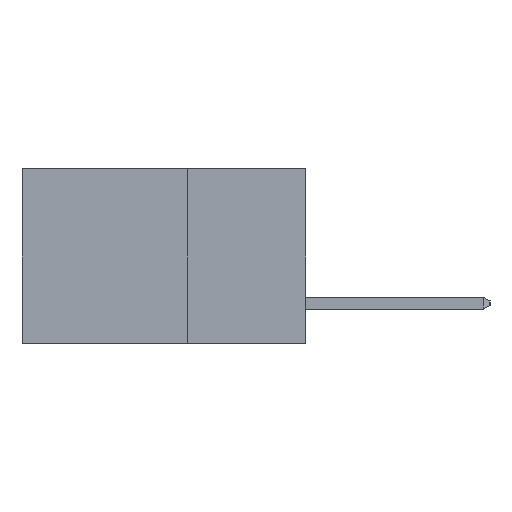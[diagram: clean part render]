
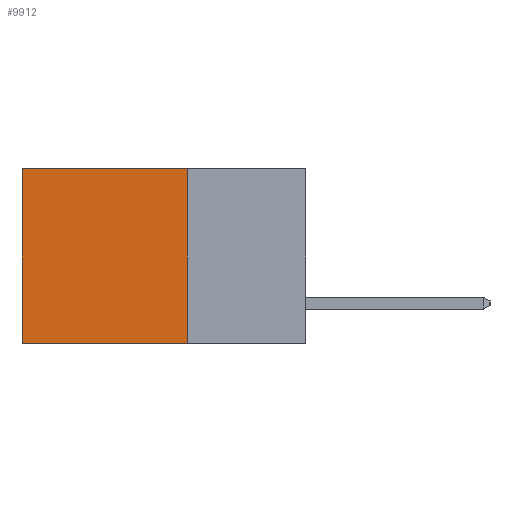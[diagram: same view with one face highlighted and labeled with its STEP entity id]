
A CAD part, left-side view. The second image highlights one B-rep face of the part: STEP entity #9912.
In plain terms, the highlighted planar face has unit normal (-1, 0, 0).
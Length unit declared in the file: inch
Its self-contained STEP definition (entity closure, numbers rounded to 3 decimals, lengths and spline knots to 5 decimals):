
#620 = LINE ( 'NONE', #13677, #1157 ) ;
#1157 = VECTOR ( 'NONE', #13656, 39.37008 ) ;
#1294 = LINE ( 'NONE', #17770, #9365 ) ;
#1515 = DIRECTION ( 'NONE',  ( 0., 1., 0. ) ) ;
#1971 = CARTESIAN_POINT ( 'NONE',  ( 0.2615, 0.6, 0. ) ) ;
#2128 = CARTESIAN_POINT ( 'NONE',  ( 0.2615, 0.25, -0.37 ) ) ;
#2547 = VERTEX_POINT ( 'NONE', #5227 ) ;
#4228 = ORIENTED_EDGE ( 'NONE', *, *, #6359, .F. ) ;
#5227 = CARTESIAN_POINT ( 'NONE',  ( 0.2615, 0.6, -0.37 ) ) ;
#5996 = VECTOR ( 'NONE', #1515, 39.37008 ) ;
#6359 = EDGE_CURVE ( 'NONE', #9627, #2547, #15925, .T. ) ;
#6627 = VERTEX_POINT ( 'NONE', #16315 ) ;
#9365 = VECTOR ( 'NONE', #17701, 39.37008 ) ;
#9627 = VERTEX_POINT ( 'NONE', #17971 ) ;
#9912 = ADVANCED_FACE ( 'NONE', ( #15839 ), #18465, .F. ) ;
#10408 = EDGE_CURVE ( 'NONE', #6627, #9627, #15329, .T. ) ;
#11313 = EDGE_CURVE ( 'NONE', #6627, #17064, #1294, .T. ) ;
#11904 = ORIENTED_EDGE ( 'NONE', *, *, #11313, .T. ) ;
#12364 = AXIS2_PLACEMENT_3D ( 'NONE', #18436, #18370, #18341 ) ;
#12371 = ORIENTED_EDGE ( 'NONE', *, *, #14330, .T. ) ;
#13656 = DIRECTION ( 'NONE',  ( 0., 0., -1. ) ) ;
#13677 = CARTESIAN_POINT ( 'NONE',  ( 0.2615, 0.6, -0.37 ) ) ;
#14330 = EDGE_CURVE ( 'NONE', #17064, #2547, #620, .T. ) ;
#14795 = EDGE_LOOP ( 'NONE', ( #12371, #4228, #17617, #11904 ) ) ;
#15329 = LINE ( 'NONE', #20101, #18571 ) ;
#15839 = FACE_OUTER_BOUND ( 'NONE', #14795, .T. ) ;
#15925 = LINE ( 'NONE', #2128, #5996 ) ;
#16315 = CARTESIAN_POINT ( 'NONE',  ( 0.2615, 0.25, 0. ) ) ;
#17064 = VERTEX_POINT ( 'NONE', #1971 ) ;
#17617 = ORIENTED_EDGE ( 'NONE', *, *, #10408, .F. ) ;
#17701 = DIRECTION ( 'NONE',  ( 0., 1., 0. ) ) ;
#17770 = CARTESIAN_POINT ( 'NONE',  ( 0.2615, 0.25, 0. ) ) ;
#17971 = CARTESIAN_POINT ( 'NONE',  ( 0.2615, 0.25, -0.37 ) ) ;
#18341 = DIRECTION ( 'NONE',  ( 0., 0., -1. ) ) ;
#18370 = DIRECTION ( 'NONE',  ( 1., 0., 0. ) ) ;
#18436 = CARTESIAN_POINT ( 'NONE',  ( 0.2615, 0.25, -0.37 ) ) ;
#18465 = PLANE ( 'NONE',  #12364 ) ;
#18571 = VECTOR ( 'NONE', #20549, 39.37008 ) ;
#20101 = CARTESIAN_POINT ( 'NONE',  ( 0.2615, 0.25, -0.37 ) ) ;
#20549 = DIRECTION ( 'NONE',  ( 0., 0., -1. ) ) ;
